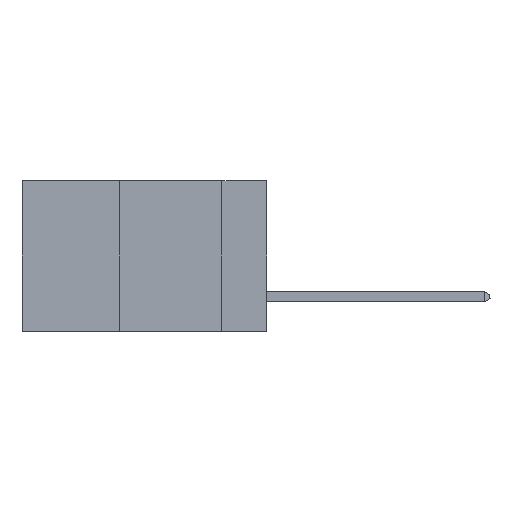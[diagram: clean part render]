
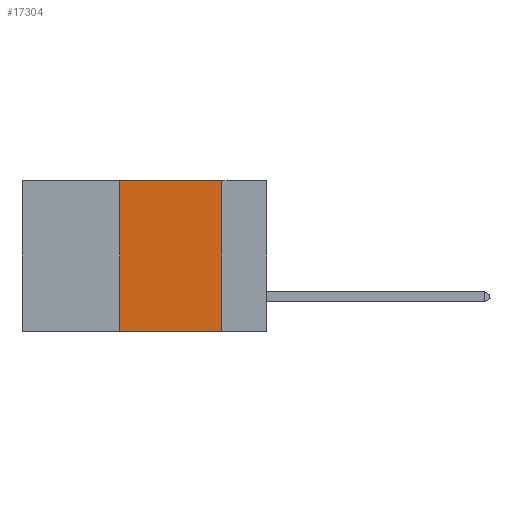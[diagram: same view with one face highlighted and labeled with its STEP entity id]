
A CAD part, left-side view. The second image highlights one B-rep face of the part: STEP entity #17304.
In plain terms, the highlighted planar face has unit normal (-1, 0, 0).
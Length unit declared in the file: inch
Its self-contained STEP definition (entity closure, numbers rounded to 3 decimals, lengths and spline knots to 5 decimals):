
#869 = DIRECTION ( 'NONE',  ( 0., 0., -1. ) ) ;
#2052 = CARTESIAN_POINT ( 'NONE',  ( 0., 0.36, -0.37 ) ) ;
#3171 = CARTESIAN_POINT ( 'NONE',  ( 0., 0.11, 0. ) ) ;
#3403 = CARTESIAN_POINT ( 'NONE',  ( 0., 0.36, 0. ) ) ;
#5013 = DIRECTION ( 'NONE',  ( 1., 0., 0. ) ) ;
#5709 = DIRECTION ( 'NONE',  ( 0., -1., 0. ) ) ;
#6234 = VERTEX_POINT ( 'NONE', #46903 ) ;
#9890 = LINE ( 'NONE', #3171, #27667 ) ;
#10570 = LINE ( 'NONE', #15445, #14114 ) ;
#12263 = VERTEX_POINT ( 'NONE', #2052 ) ;
#14114 = VECTOR ( 'NONE', #33984, 39.37008 ) ;
#15081 = EDGE_CURVE ( 'NONE', #16226, #6234, #42613, .T. ) ;
#15324 = AXIS2_PLACEMENT_3D ( 'NONE', #34539, #5013, #869 ) ;
#15445 = CARTESIAN_POINT ( 'NONE',  ( 0., 0.6, -0.37 ) ) ;
#15877 = EDGE_CURVE ( 'NONE', #12263, #46964, #10570, .T. ) ;
#16226 = VERTEX_POINT ( 'NONE', #3403 ) ;
#17304 = ADVANCED_FACE ( 'NONE', ( #22346 ), #42108, .F. ) ;
#17973 = DIRECTION ( 'NONE',  ( 0., 0., 1. ) ) ;
#18748 = DIRECTION ( 'NONE',  ( 0., 0., -1. ) ) ;
#21457 = CARTESIAN_POINT ( 'NONE',  ( 0., 0.6, 0. ) ) ;
#21545 = EDGE_LOOP ( 'NONE', ( #27109, #48110, #36653, #37094 ) ) ;
#22346 = FACE_OUTER_BOUND ( 'NONE', #21545, .T. ) ;
#25420 = CARTESIAN_POINT ( 'NONE',  ( 0., 0.36, 0. ) ) ;
#26816 = CARTESIAN_POINT ( 'NONE',  ( 0., 0.11, -0.37 ) ) ;
#27109 = ORIENTED_EDGE ( 'NONE', *, *, #39509, .F. ) ;
#27667 = VECTOR ( 'NONE', #18748, 39.37008 ) ;
#29619 = VECTOR ( 'NONE', #5709, 39.37008 ) ;
#33984 = DIRECTION ( 'NONE',  ( 0., -1., 0. ) ) ;
#34539 = CARTESIAN_POINT ( 'NONE',  ( 0., 0.6, 0. ) ) ;
#36588 = VECTOR ( 'NONE', #17973, 39.37008 ) ;
#36653 = ORIENTED_EDGE ( 'NONE', *, *, #47752, .F. ) ;
#37094 = ORIENTED_EDGE ( 'NONE', *, *, #15877, .T. ) ;
#39509 = EDGE_CURVE ( 'NONE', #6234, #46964, #9890, .T. ) ;
#42108 = PLANE ( 'NONE',  #15324 ) ;
#42613 = LINE ( 'NONE', #21457, #29619 ) ;
#46006 = LINE ( 'NONE', #25420, #36588 ) ;
#46903 = CARTESIAN_POINT ( 'NONE',  ( 0., 0.11, 0. ) ) ;
#46964 = VERTEX_POINT ( 'NONE', #26816 ) ;
#47752 = EDGE_CURVE ( 'NONE', #12263, #16226, #46006, .T. ) ;
#48110 = ORIENTED_EDGE ( 'NONE', *, *, #15081, .F. ) ;
